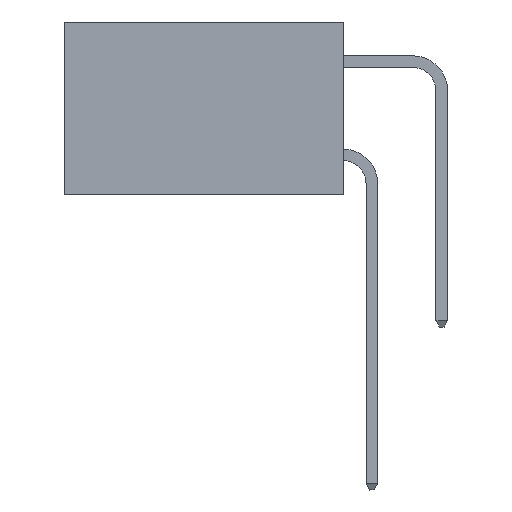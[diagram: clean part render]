
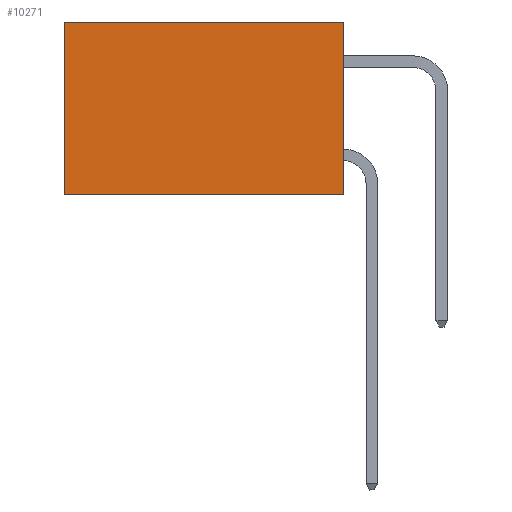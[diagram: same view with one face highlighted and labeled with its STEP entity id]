
A CAD part, left-side view. The second image highlights one B-rep face of the part: STEP entity #10271.
In plain terms, the highlighted planar face has unit normal (-1, 0, 0).
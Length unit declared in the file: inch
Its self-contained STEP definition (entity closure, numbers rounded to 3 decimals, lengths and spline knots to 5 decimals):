
#668 = VERTEX_POINT ( 'NONE', #6148 ) ;
#735 = EDGE_CURVE ( 'NONE', #25111, #668, #9459, .T. ) ;
#931 = CARTESIAN_POINT ( 'NONE',  ( 0.2615, 0., -0.37 ) ) ;
#3170 = DIRECTION ( 'NONE',  ( 1., 0., 0. ) ) ;
#4073 = CARTESIAN_POINT ( 'NONE',  ( 0.2615, 0.6, 0. ) ) ;
#5727 = CARTESIAN_POINT ( 'NONE',  ( 0.2615, 0.6, -0.37 ) ) ;
#6018 = DIRECTION ( 'NONE',  ( 0., 0., -1. ) ) ;
#6131 = CARTESIAN_POINT ( 'NONE',  ( 0.2615, 0., 0. ) ) ;
#6148 = CARTESIAN_POINT ( 'NONE',  ( 0.2615, 0.6, -0.37 ) ) ;
#6375 = ORIENTED_EDGE ( 'NONE', *, *, #12802, .F. ) ;
#8226 = AXIS2_PLACEMENT_3D ( 'NONE', #931, #3170, #18365 ) ;
#9459 = LINE ( 'NONE', #5727, #15182 ) ;
#10271 = ADVANCED_FACE ( 'NONE', ( #25124 ), #14039, .F. ) ;
#10792 = CARTESIAN_POINT ( 'NONE',  ( 0.2615, 0., -0.37 ) ) ;
#10923 = VECTOR ( 'NONE', #25772, 39.37008 ) ;
#11685 = DIRECTION ( 'NONE',  ( 0., 0., -1. ) ) ;
#12802 = EDGE_CURVE ( 'NONE', #13792, #668, #16925, .T. ) ;
#13306 = ORIENTED_EDGE ( 'NONE', *, *, #735, .T. ) ;
#13792 = VERTEX_POINT ( 'NONE', #26794 ) ;
#14039 = PLANE ( 'NONE',  #8226 ) ;
#14419 = EDGE_CURVE ( 'NONE', #27631, #25111, #18654, .T. ) ;
#15063 = CARTESIAN_POINT ( 'NONE',  ( 0.2615, 0., 0. ) ) ;
#15182 = VECTOR ( 'NONE', #6018, 39.37008 ) ;
#16064 = EDGE_CURVE ( 'NONE', #27631, #13792, #25985, .T. ) ;
#16925 = LINE ( 'NONE', #10792, #22638 ) ;
#18101 = CARTESIAN_POINT ( 'NONE',  ( 0.2615, 0., -0.37 ) ) ;
#18365 = DIRECTION ( 'NONE',  ( 0., 0., -1. ) ) ;
#18654 = LINE ( 'NONE', #15063, #10923 ) ;
#19224 = ORIENTED_EDGE ( 'NONE', *, *, #16064, .F. ) ;
#20301 = VECTOR ( 'NONE', #11685, 39.37008 ) ;
#21018 = EDGE_LOOP ( 'NONE', ( #13306, #6375, #19224, #21184 ) ) ;
#21184 = ORIENTED_EDGE ( 'NONE', *, *, #14419, .T. ) ;
#22638 = VECTOR ( 'NONE', #23755, 39.37008 ) ;
#23755 = DIRECTION ( 'NONE',  ( 0., 1., 0. ) ) ;
#25111 = VERTEX_POINT ( 'NONE', #4073 ) ;
#25124 = FACE_OUTER_BOUND ( 'NONE', #21018, .T. ) ;
#25772 = DIRECTION ( 'NONE',  ( 0., 1., 0. ) ) ;
#25985 = LINE ( 'NONE', #18101, #20301 ) ;
#26794 = CARTESIAN_POINT ( 'NONE',  ( 0.2615, 0., -0.37 ) ) ;
#27631 = VERTEX_POINT ( 'NONE', #6131 ) ;
